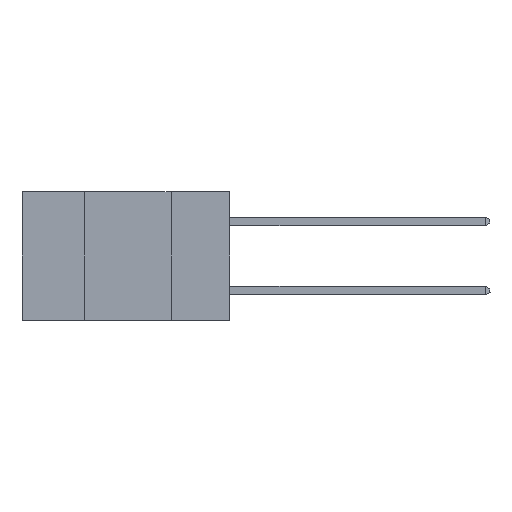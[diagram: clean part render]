
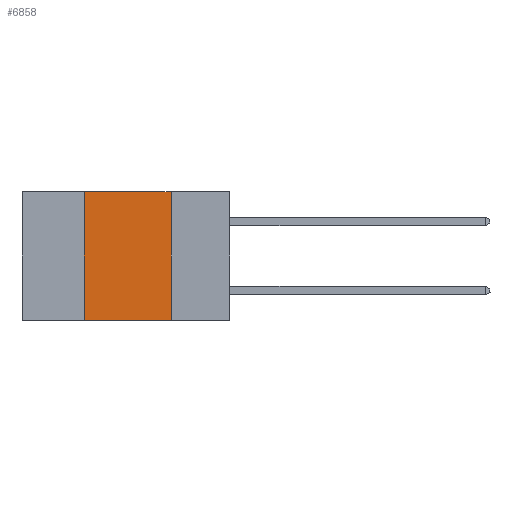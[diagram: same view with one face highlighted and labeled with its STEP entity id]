
A CAD part, left-side view. The second image highlights one B-rep face of the part: STEP entity #6858.
In plain terms, the highlighted planar face has unit normal (-1, 0, 0).
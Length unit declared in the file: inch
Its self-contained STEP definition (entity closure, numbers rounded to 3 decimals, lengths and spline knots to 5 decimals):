
#2324 = LINE ( 'NONE', #12832, #7602 ) ;
#2432 = LINE ( 'NONE', #30741, #15289 ) ;
#2579 = ORIENTED_EDGE ( 'NONE', *, *, #17194, .F. ) ;
#4233 = DIRECTION ( 'NONE',  ( 0., 0., -1. ) ) ;
#4493 = FACE_OUTER_BOUND ( 'NONE', #17183, .T. ) ;
#5291 = DIRECTION ( 'NONE',  ( 0., -1., 0. ) ) ;
#6029 = DIRECTION ( 'NONE',  ( 0., 0., -1. ) ) ;
#6858 = ADVANCED_FACE ( 'NONE', ( #4493 ), #32192, .F. ) ;
#7602 = VECTOR ( 'NONE', #17633, 39.37008 ) ;
#8209 = CARTESIAN_POINT ( 'NONE',  ( 0., 0.42, 0. ) ) ;
#8417 = VERTEX_POINT ( 'NONE', #27731 ) ;
#9273 = EDGE_CURVE ( 'NONE', #25357, #8417, #24323, .T. ) ;
#12255 = AXIS2_PLACEMENT_3D ( 'NONE', #16985, #19573, #4233 ) ;
#12370 = VECTOR ( 'NONE', #24718, 39.37008 ) ;
#12832 = CARTESIAN_POINT ( 'NONE',  ( 0., 0.42, 0. ) ) ;
#13064 = CARTESIAN_POINT ( 'NONE',  ( 0., 0.42, -0.37 ) ) ;
#15289 = VECTOR ( 'NONE', #5291, 39.37008 ) ;
#16714 = VERTEX_POINT ( 'NONE', #28780 ) ;
#16985 = CARTESIAN_POINT ( 'NONE',  ( 0., 0.6, 0. ) ) ;
#17183 = EDGE_LOOP ( 'NONE', ( #21387, #23474, #2579, #27747 ) ) ;
#17194 = EDGE_CURVE ( 'NONE', #17253, #25357, #2324, .T. ) ;
#17253 = VERTEX_POINT ( 'NONE', #13064 ) ;
#17633 = DIRECTION ( 'NONE',  ( 0., 0., 1. ) ) ;
#19573 = DIRECTION ( 'NONE',  ( 1., 0., 0. ) ) ;
#21368 = CARTESIAN_POINT ( 'NONE',  ( 0., 0.17, 0. ) ) ;
#21387 = ORIENTED_EDGE ( 'NONE', *, *, #28771, .F. ) ;
#22027 = VECTOR ( 'NONE', #6029, 39.37008 ) ;
#22151 = CARTESIAN_POINT ( 'NONE',  ( 0., 0.6, 0. ) ) ;
#23474 = ORIENTED_EDGE ( 'NONE', *, *, #9273, .F. ) ;
#24323 = LINE ( 'NONE', #22151, #12370 ) ;
#24694 = EDGE_CURVE ( 'NONE', #17253, #16714, #2432, .T. ) ;
#24718 = DIRECTION ( 'NONE',  ( 0., -1., 0. ) ) ;
#25357 = VERTEX_POINT ( 'NONE', #8209 ) ;
#27731 = CARTESIAN_POINT ( 'NONE',  ( 0., 0.17, 0. ) ) ;
#27747 = ORIENTED_EDGE ( 'NONE', *, *, #24694, .T. ) ;
#28001 = LINE ( 'NONE', #21368, #22027 ) ;
#28771 = EDGE_CURVE ( 'NONE', #8417, #16714, #28001, .T. ) ;
#28780 = CARTESIAN_POINT ( 'NONE',  ( 0., 0.17, -0.37 ) ) ;
#30741 = CARTESIAN_POINT ( 'NONE',  ( 0., 0.6, -0.37 ) ) ;
#32192 = PLANE ( 'NONE',  #12255 ) ;
